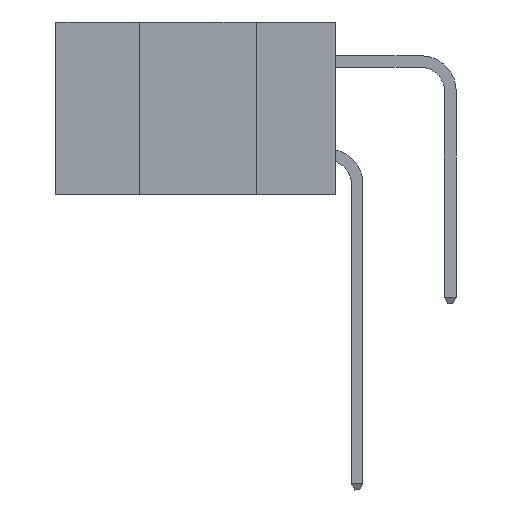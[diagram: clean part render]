
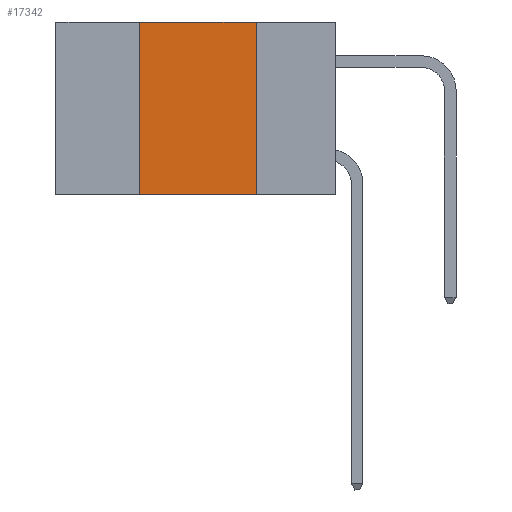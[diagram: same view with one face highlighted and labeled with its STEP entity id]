
A CAD part, left-side view. The second image highlights one B-rep face of the part: STEP entity #17342.
In plain terms, the highlighted planar face has unit normal (-1, 0, 0).
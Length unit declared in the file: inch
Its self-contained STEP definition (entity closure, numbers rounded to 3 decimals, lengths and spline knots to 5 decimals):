
#500 = CARTESIAN_POINT ( 'NONE',  ( 0., 0.6, 0. ) ) ;
#1206 = DIRECTION ( 'NONE',  ( 0., -1., 0. ) ) ;
#1427 = DIRECTION ( 'NONE',  ( 0., -1., 0. ) ) ;
#2002 = VERTEX_POINT ( 'NONE', #5241 ) ;
#3783 = VECTOR ( 'NONE', #1206, 39.37008 ) ;
#5058 = EDGE_CURVE ( 'NONE', #16108, #2002, #19232, .T. ) ;
#5241 = CARTESIAN_POINT ( 'NONE',  ( 0., 0.42, 0. ) ) ;
#5263 = VERTEX_POINT ( 'NONE', #6115 ) ;
#6115 = CARTESIAN_POINT ( 'NONE',  ( 0., 0.17, -0.37 ) ) ;
#6210 = CARTESIAN_POINT ( 'NONE',  ( 0., 0.17, 0. ) ) ;
#7027 = EDGE_CURVE ( 'NONE', #2002, #16917, #18142, .T. ) ;
#7150 = VECTOR ( 'NONE', #1427, 39.37008 ) ;
#7500 = DIRECTION ( 'NONE',  ( 1., 0., 0. ) ) ;
#8482 = ORIENTED_EDGE ( 'NONE', *, *, #5058, .F. ) ;
#8567 = PLANE ( 'NONE',  #13148 ) ;
#8906 = FACE_OUTER_BOUND ( 'NONE', #21198, .T. ) ;
#9936 = CARTESIAN_POINT ( 'NONE',  ( 0., 0.42, -0.37 ) ) ;
#10380 = VECTOR ( 'NONE', #15771, 39.37008 ) ;
#10882 = LINE ( 'NONE', #17855, #3783 ) ;
#11956 = EDGE_CURVE ( 'NONE', #16917, #5263, #12167, .T. ) ;
#12167 = LINE ( 'NONE', #17308, #10380 ) ;
#12944 = VECTOR ( 'NONE', #14322, 39.37008 ) ;
#13148 = AXIS2_PLACEMENT_3D ( 'NONE', #500, #7500, #19510 ) ;
#14141 = EDGE_CURVE ( 'NONE', #16108, #5263, #10882, .T. ) ;
#14166 = ORIENTED_EDGE ( 'NONE', *, *, #7027, .F. ) ;
#14322 = DIRECTION ( 'NONE',  ( 0., 0., 1. ) ) ;
#14347 = ORIENTED_EDGE ( 'NONE', *, *, #11956, .F. ) ;
#15079 = ORIENTED_EDGE ( 'NONE', *, *, #14141, .T. ) ;
#15771 = DIRECTION ( 'NONE',  ( 0., 0., -1. ) ) ;
#15909 = CARTESIAN_POINT ( 'NONE',  ( 0., 0.42, 0. ) ) ;
#16108 = VERTEX_POINT ( 'NONE', #9936 ) ;
#16917 = VERTEX_POINT ( 'NONE', #6210 ) ;
#17308 = CARTESIAN_POINT ( 'NONE',  ( 0., 0.17, 0. ) ) ;
#17342 = ADVANCED_FACE ( 'NONE', ( #8906 ), #8567, .F. ) ;
#17855 = CARTESIAN_POINT ( 'NONE',  ( 0., 0.6, -0.37 ) ) ;
#18142 = LINE ( 'NONE', #20101, #7150 ) ;
#19232 = LINE ( 'NONE', #15909, #12944 ) ;
#19510 = DIRECTION ( 'NONE',  ( 0., 0., -1. ) ) ;
#20101 = CARTESIAN_POINT ( 'NONE',  ( 0., 0.6, 0. ) ) ;
#21198 = EDGE_LOOP ( 'NONE', ( #14347, #14166, #8482, #15079 ) ) ;
